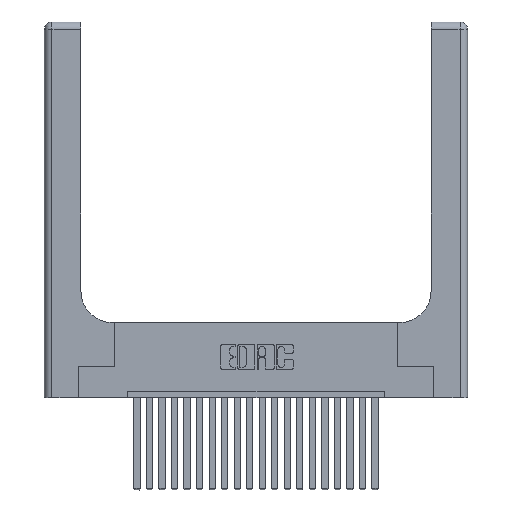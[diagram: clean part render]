
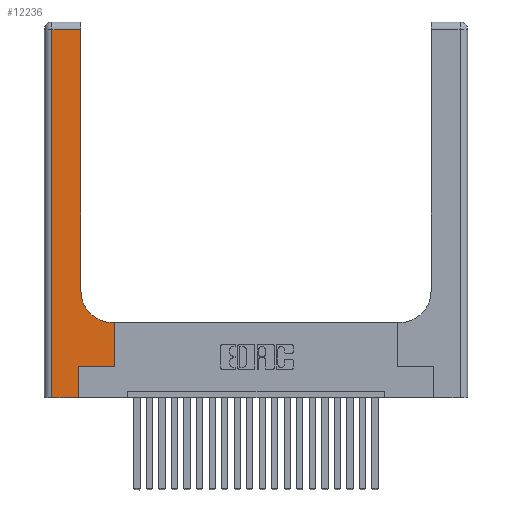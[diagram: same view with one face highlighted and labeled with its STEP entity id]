
A CAD part, top view. The second image highlights one B-rep face of the part: STEP entity #12236.
In plain terms, the highlighted planar face has unit normal (0, 0, 1).
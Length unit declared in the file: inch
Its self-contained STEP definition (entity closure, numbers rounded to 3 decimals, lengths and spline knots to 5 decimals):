
#90 = EDGE_CURVE ( 'NONE', #22160, #17144, #10728, .T. ) ;
#275 = CARTESIAN_POINT ( 'NONE',  ( 0.269, 0., 0.37 ) ) ;
#408 = CARTESIAN_POINT ( 'NONE',  ( 0.2915, 0.85, 0.37 ) ) ;
#866 = LINE ( 'NONE', #275, #9772 ) ;
#977 = VERTEX_POINT ( 'NONE', #15435 ) ;
#1510 = AXIS2_PLACEMENT_3D ( 'NONE', #8283, #4707, #10248 ) ;
#1560 = AXIS2_PLACEMENT_3D ( 'NONE', #19831, #16564, #14554 ) ;
#1704 = CARTESIAN_POINT ( 'NONE',  ( 0.269, 0.25, 0.37 ) ) ;
#1714 = DIRECTION ( 'NONE',  ( 0., 1., 0. ) ) ;
#1924 = EDGE_CURVE ( 'NONE', #13619, #22160, #866, .T. ) ;
#1946 = CARTESIAN_POINT ( 'NONE',  ( 0.06, 3., 0.37 ) ) ;
#2220 = CARTESIAN_POINT ( 'NONE',  ( 0.5585, 0.25, 0.37 ) ) ;
#2600 = VERTEX_POINT ( 'NONE', #17567 ) ;
#3009 = VECTOR ( 'NONE', #11103, 39.37008 ) ;
#3799 = CARTESIAN_POINT ( 'NONE',  ( 0.2915, 0.6, 0.37 ) ) ;
#3981 = LINE ( 'NONE', #1946, #11503 ) ;
#4277 = ORIENTED_EDGE ( 'NONE', *, *, #15298, .T. ) ;
#4707 = DIRECTION ( 'NONE',  ( 0., 0., -1. ) ) ;
#5533 = DIRECTION ( 'NONE',  ( 0., -1., 0. ) ) ;
#5749 = EDGE_LOOP ( 'NONE', ( #7152, #13175, #10480, #9769, #10190, #11508, #12706, #7568, #4277 ) ) ;
#5814 = CIRCLE ( 'NONE', #1510, 0.25 ) ;
#6865 = VERTEX_POINT ( 'NONE', #408 ) ;
#7152 = ORIENTED_EDGE ( 'NONE', *, *, #14303, .T. ) ;
#7380 = PLANE ( 'NONE',  #1560 ) ;
#7568 = ORIENTED_EDGE ( 'NONE', *, *, #15531, .T. ) ;
#7647 = CARTESIAN_POINT ( 'NONE',  ( 0.5585, 0.6, 0.37 ) ) ;
#7679 = VERTEX_POINT ( 'NONE', #16582 ) ;
#7809 = FACE_OUTER_BOUND ( 'NONE', #5749, .T. ) ;
#8283 = CARTESIAN_POINT ( 'NONE',  ( 0.5415, 0.85, 0.37 ) ) ;
#8372 = CARTESIAN_POINT ( 'NONE',  ( 0., 0., 0.37 ) ) ;
#9132 = CARTESIAN_POINT ( 'NONE',  ( 0.269, 0.25, 0.37 ) ) ;
#9550 = VERTEX_POINT ( 'NONE', #21612 ) ;
#9769 = ORIENTED_EDGE ( 'NONE', *, *, #12484, .T. ) ;
#9772 = VECTOR ( 'NONE', #12715, 39.37008 ) ;
#10190 = ORIENTED_EDGE ( 'NONE', *, *, #1924, .T. ) ;
#10248 = DIRECTION ( 'NONE',  ( 1., 0., 0. ) ) ;
#10314 = VECTOR ( 'NONE', #18944, 39.37008 ) ;
#10480 = ORIENTED_EDGE ( 'NONE', *, *, #10623, .T. ) ;
#10481 = CARTESIAN_POINT ( 'NONE',  ( 0.269, 0., 0.37 ) ) ;
#10623 = EDGE_CURVE ( 'NONE', #7679, #977, #3981, .T. ) ;
#10728 = LINE ( 'NONE', #1704, #19628 ) ;
#11103 = DIRECTION ( 'NONE',  ( -1., 0., 0. ) ) ;
#11503 = VECTOR ( 'NONE', #5533, 39.37008 ) ;
#11508 = ORIENTED_EDGE ( 'NONE', *, *, #90, .T. ) ;
#12199 = LINE ( 'NONE', #3799, #3009 ) ;
#12236 = ADVANCED_FACE ( 'NONE', ( #7809 ), #7380, .F. ) ;
#12405 = CARTESIAN_POINT ( 'NONE',  ( 0.5585, 0.25, 0.37 ) ) ;
#12484 = EDGE_CURVE ( 'NONE', #977, #13619, #15051, .T. ) ;
#12706 = ORIENTED_EDGE ( 'NONE', *, *, #17638, .T. ) ;
#12715 = DIRECTION ( 'NONE',  ( 0., 1., 0. ) ) ;
#13175 = ORIENTED_EDGE ( 'NONE', *, *, #13304, .T. ) ;
#13304 = EDGE_CURVE ( 'NONE', #9550, #7679, #23022, .T. ) ;
#13619 = VERTEX_POINT ( 'NONE', #10481 ) ;
#14303 = EDGE_CURVE ( 'NONE', #6865, #9550, #21450, .T. ) ;
#14554 = DIRECTION ( 'NONE',  ( -1., 0., 0. ) ) ;
#15051 = LINE ( 'NONE', #8372, #10314 ) ;
#15298 = EDGE_CURVE ( 'NONE', #2600, #6865, #5814, .T. ) ;
#15435 = CARTESIAN_POINT ( 'NONE',  ( 0.06, 0., 0.37 ) ) ;
#15531 = EDGE_CURVE ( 'NONE', #16399, #2600, #12199, .T. ) ;
#15624 = VECTOR ( 'NONE', #22601, 39.37008 ) ;
#16399 = VERTEX_POINT ( 'NONE', #7647 ) ;
#16564 = DIRECTION ( 'NONE',  ( 0., 0., -1. ) ) ;
#16582 = CARTESIAN_POINT ( 'NONE',  ( 0.06, 2.94, 0.37 ) ) ;
#16898 = LINE ( 'NONE', #12405, #21876 ) ;
#17144 = VERTEX_POINT ( 'NONE', #2220 ) ;
#17567 = CARTESIAN_POINT ( 'NONE',  ( 0.5415, 0.6, 0.37 ) ) ;
#17638 = EDGE_CURVE ( 'NONE', #17144, #16399, #16898, .T. ) ;
#18944 = DIRECTION ( 'NONE',  ( 1., 0., 0. ) ) ;
#19522 = DIRECTION ( 'NONE',  ( 1., 0., 0. ) ) ;
#19628 = VECTOR ( 'NONE', #19522, 39.37008 ) ;
#19831 = CARTESIAN_POINT ( 'NONE',  ( 0., 3., 0.37 ) ) ;
#19947 = VECTOR ( 'NONE', #21907, 39.37008 ) ;
#21450 = LINE ( 'NONE', #22443, #15624 ) ;
#21612 = CARTESIAN_POINT ( 'NONE',  ( 0.2915, 2.94, 0.37 ) ) ;
#21876 = VECTOR ( 'NONE', #1714, 39.37008 ) ;
#21907 = DIRECTION ( 'NONE',  ( -1., 0., 0. ) ) ;
#21972 = CARTESIAN_POINT ( 'NONE',  ( 0., 2.94, 0.37 ) ) ;
#22160 = VERTEX_POINT ( 'NONE', #9132 ) ;
#22443 = CARTESIAN_POINT ( 'NONE',  ( 0.2915, 3., 0.37 ) ) ;
#22601 = DIRECTION ( 'NONE',  ( 0., 1., 0. ) ) ;
#23022 = LINE ( 'NONE', #21972, #19947 ) ;
